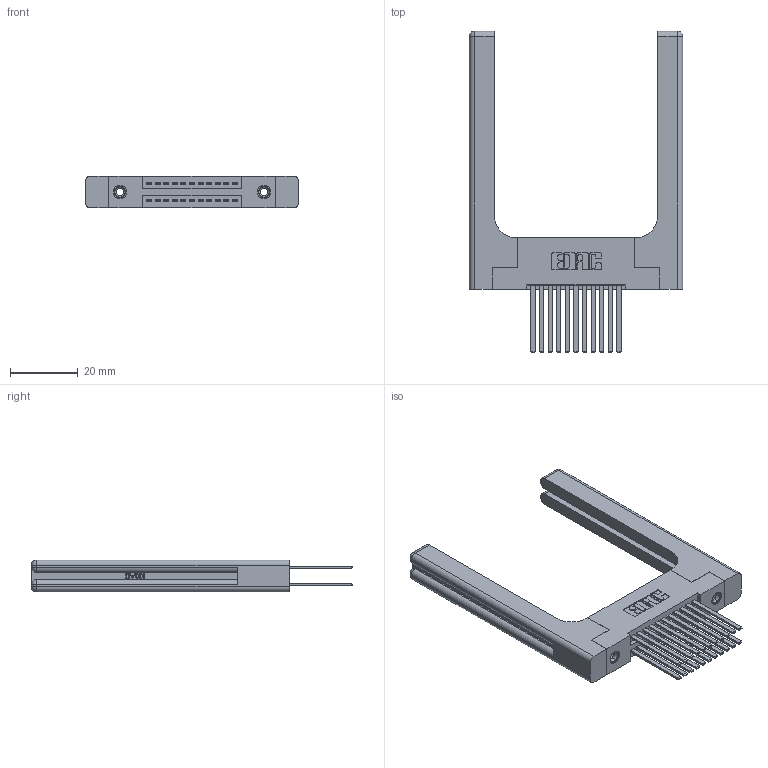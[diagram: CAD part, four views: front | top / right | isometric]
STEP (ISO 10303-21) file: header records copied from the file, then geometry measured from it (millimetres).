
FILE_DESCRIPTION (( 'STEP AP203' ), '1' );
FILE_NAME ('395-022-544-258.STEP', '2019-10-15T23:21:49', ( '' ), ( '' ), 'SwSTEP 2.0', 'SolidWorks 2016', '' );
FILE_SCHEMA (( 'CONFIG_CONTROL_DESIGN' ));
Length unit declared in the file: inch
Products named in the file (5): 345-250-001_345-250-001-102; 345-220-058_345-220-058; 395-022-544-258; 345 Part_Flush Mounting Lugs - 0.156 Dia-TH; 345-292-001_345-293-144
Assembly tree (27 placements, depth 2):
  395-022-544-258
    345 Part_Flush Mounting Lugs - 0.156 Dia-TH
    345-292-001_345-293-144  x22
    345-250-001_345-250-001-102  x2
    345-220-058_345-220-058  x2
Bounding box: 62.97 x 94.92 x 9.4 mm (x, y, z)
Volume: 14612.4 mm3; surface area: 14434.3 mm2
Topology: 27 solids, 27 shells, 1350 faces, 3889 edges, 2542 vertices
Faces by surface type: plane 866, cylinder 424, bspline 36, cone 12, sphere 8, torus 4
Entity records: 17802 total; most frequent: CARTESIAN_POINT 4005, ORIENTED_EDGE 2736, DIRECTION 2500, EDGE_CURVE 1368, VECTOR 1104, LINE 1104, VERTEX_POINT 902, AXIS2_PLACEMENT_3D 698
